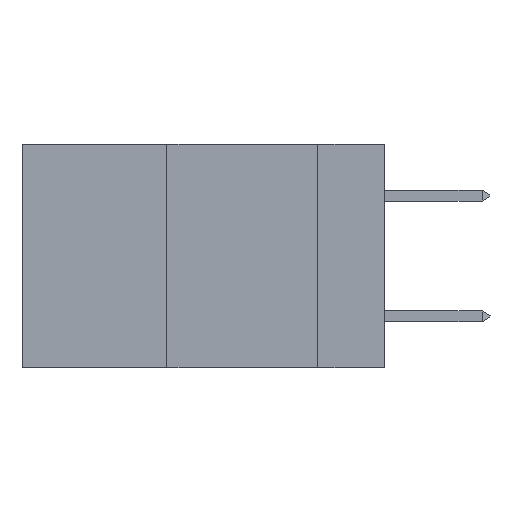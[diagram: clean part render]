
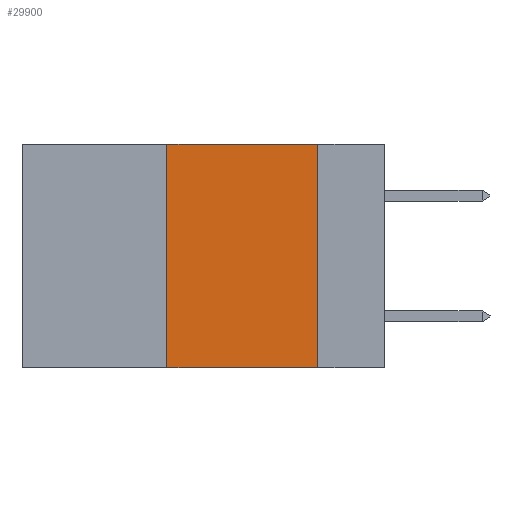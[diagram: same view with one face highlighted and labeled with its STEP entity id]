
A CAD part, left-side view. The second image highlights one B-rep face of the part: STEP entity #29900.
In plain terms, the highlighted planar face has unit normal (-1, 0, 0).
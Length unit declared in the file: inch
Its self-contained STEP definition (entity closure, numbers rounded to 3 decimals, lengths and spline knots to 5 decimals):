
#3731 = VERTEX_POINT ( 'NONE', #27008 ) ;
#4005 = CARTESIAN_POINT ( 'NONE',  ( 0., 0.6, 0. ) ) ;
#4208 = VERTEX_POINT ( 'NONE', #12384 ) ;
#4399 = VECTOR ( 'NONE', #19011, 39.37008 ) ;
#5450 = ORIENTED_EDGE ( 'NONE', *, *, #7761, .F. ) ;
#5677 = EDGE_LOOP ( 'NONE', ( #7392, #5450, #9632, #30382 ) ) ;
#5679 = PLANE ( 'NONE',  #29803 ) ;
#6978 = LINE ( 'NONE', #13931, #15566 ) ;
#7392 = ORIENTED_EDGE ( 'NONE', *, *, #29141, .F. ) ;
#7614 = LINE ( 'NONE', #16877, #4399 ) ;
#7761 = EDGE_CURVE ( 'NONE', #13400, #3731, #7614, .T. ) ;
#8315 = EDGE_CURVE ( 'NONE', #4208, #22954, #19727, .T. ) ;
#8966 = CARTESIAN_POINT ( 'NONE',  ( 0., 0.36, 0. ) ) ;
#9632 = ORIENTED_EDGE ( 'NONE', *, *, #21214, .F. ) ;
#12360 = VECTOR ( 'NONE', #15464, 39.37008 ) ;
#12384 = CARTESIAN_POINT ( 'NONE',  ( 0., 0.36, -0.37 ) ) ;
#13400 = VERTEX_POINT ( 'NONE', #20580 ) ;
#13399 = DIRECTION ( 'NONE',  ( 1., 0., 0. ) ) ;
#13931 = CARTESIAN_POINT ( 'NONE',  ( 0., 0.11, 0. ) ) ;
#14392 = DIRECTION ( 'NONE',  ( 0., 0., -1. ) ) ;
#15464 = DIRECTION ( 'NONE',  ( 0., 0., 1. ) ) ;
#15566 = VECTOR ( 'NONE', #14392, 39.37008 ) ;
#16877 = CARTESIAN_POINT ( 'NONE',  ( 0., 0.6, 0. ) ) ;
#17433 = CARTESIAN_POINT ( 'NONE',  ( 0., 0.6, -0.37 ) ) ;
#17857 = VECTOR ( 'NONE', #19428, 39.37008 ) ;
#17996 = FACE_OUTER_BOUND ( 'NONE', #5677, .T. ) ;
#19011 = DIRECTION ( 'NONE',  ( 0., -1., 0. ) ) ;
#19428 = DIRECTION ( 'NONE',  ( 0., -1., 0. ) ) ;
#19727 = LINE ( 'NONE', #17433, #17857 ) ;
#20580 = CARTESIAN_POINT ( 'NONE',  ( 0., 0.36, 0. ) ) ;
#21214 = EDGE_CURVE ( 'NONE', #4208, #13400, #27269, .T. ) ;
#22954 = VERTEX_POINT ( 'NONE', #29714 ) ;
#27008 = CARTESIAN_POINT ( 'NONE',  ( 0., 0.11, 0. ) ) ;
#27269 = LINE ( 'NONE', #8966, #12360 ) ;
#29141 = EDGE_CURVE ( 'NONE', #3731, #22954, #6978, .T. ) ;
#29714 = CARTESIAN_POINT ( 'NONE',  ( 0., 0.11, -0.37 ) ) ;
#29803 = AXIS2_PLACEMENT_3D ( 'NONE', #4005, #13399, #29840 ) ;
#29840 = DIRECTION ( 'NONE',  ( 0., 0., -1. ) ) ;
#29900 = ADVANCED_FACE ( 'NONE', ( #17996 ), #5679, .F. ) ;
#30382 = ORIENTED_EDGE ( 'NONE', *, *, #8315, .T. ) ;
